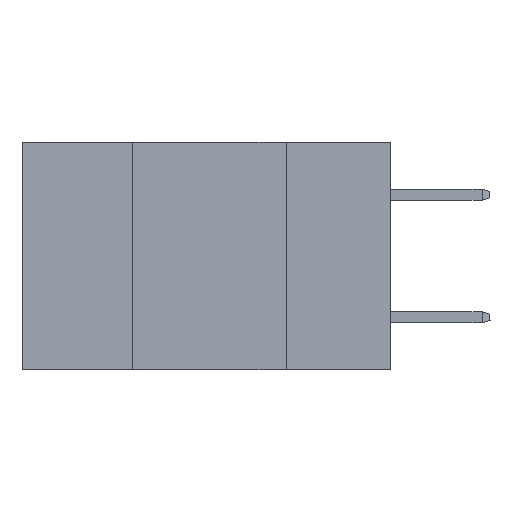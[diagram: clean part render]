
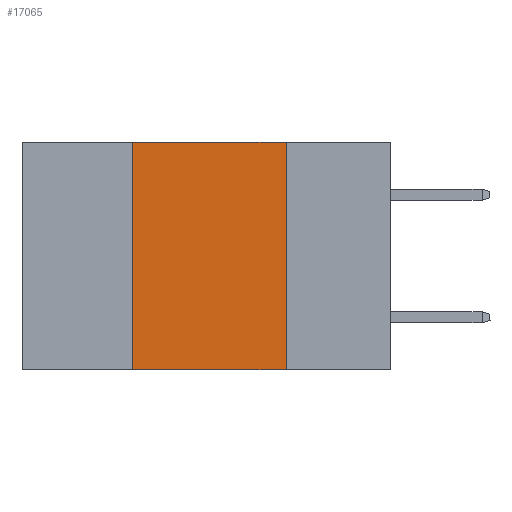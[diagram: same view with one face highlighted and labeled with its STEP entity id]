
A CAD part, left-side view. The second image highlights one B-rep face of the part: STEP entity #17065.
In plain terms, the highlighted planar face has unit normal (-1, 0, 0).
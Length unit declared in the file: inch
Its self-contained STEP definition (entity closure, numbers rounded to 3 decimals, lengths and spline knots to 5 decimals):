
#705 = EDGE_CURVE ( 'NONE', #16371, #19525, #12678, .T. ) ;
#773 = EDGE_CURVE ( 'NONE', #7617, #10101, #20423, .T. ) ;
#986 = DIRECTION ( 'NONE',  ( 0., -1., 0. ) ) ;
#1104 = ORIENTED_EDGE ( 'NONE', *, *, #20048, .F. ) ;
#1252 = VECTOR ( 'NONE', #986, 39.37008 ) ;
#1673 = CARTESIAN_POINT ( 'NONE',  ( 0., 0.6, -0.37 ) ) ;
#3305 = VECTOR ( 'NONE', #12870, 39.37008 ) ;
#3714 = CARTESIAN_POINT ( 'NONE',  ( 0., 0.6, 0. ) ) ;
#4574 = VECTOR ( 'NONE', #19453, 39.37008 ) ;
#4777 = FACE_OUTER_BOUND ( 'NONE', #10656, .T. ) ;
#5422 = DIRECTION ( 'NONE',  ( 0., 0., -1. ) ) ;
#7617 = VERTEX_POINT ( 'NONE', #8149 ) ;
#7718 = LINE ( 'NONE', #26572, #16099 ) ;
#7779 = ORIENTED_EDGE ( 'NONE', *, *, #705, .F. ) ;
#8149 = CARTESIAN_POINT ( 'NONE',  ( 0., 0.42, -0.37 ) ) ;
#8180 = CARTESIAN_POINT ( 'NONE',  ( 0., 0.17, 0. ) ) ;
#8745 = AXIS2_PLACEMENT_3D ( 'NONE', #3714, #10042, #20857 ) ;
#9010 = LINE ( 'NONE', #23450, #3305 ) ;
#9023 = CARTESIAN_POINT ( 'NONE',  ( 0., 0.42, 0. ) ) ;
#10042 = DIRECTION ( 'NONE',  ( 1., 0., 0. ) ) ;
#10101 = VERTEX_POINT ( 'NONE', #25231 ) ;
#10339 = ORIENTED_EDGE ( 'NONE', *, *, #773, .T. ) ;
#10444 = EDGE_CURVE ( 'NONE', #19525, #10101, #7718, .T. ) ;
#10656 = EDGE_LOOP ( 'NONE', ( #11069, #7779, #1104, #10339 ) ) ;
#11069 = ORIENTED_EDGE ( 'NONE', *, *, #10444, .F. ) ;
#11804 = CARTESIAN_POINT ( 'NONE',  ( 0., 0.6, 0. ) ) ;
#12678 = LINE ( 'NONE', #11804, #1252 ) ;
#12870 = DIRECTION ( 'NONE',  ( 0., 0., 1. ) ) ;
#16099 = VECTOR ( 'NONE', #5422, 39.37008 ) ;
#16371 = VERTEX_POINT ( 'NONE', #9023 ) ;
#16568 = PLANE ( 'NONE',  #8745 ) ;
#17065 = ADVANCED_FACE ( 'NONE', ( #4777 ), #16568, .F. ) ;
#19453 = DIRECTION ( 'NONE',  ( 0., -1., 0. ) ) ;
#19525 = VERTEX_POINT ( 'NONE', #8180 ) ;
#20048 = EDGE_CURVE ( 'NONE', #7617, #16371, #9010, .T. ) ;
#20423 = LINE ( 'NONE', #1673, #4574 ) ;
#20857 = DIRECTION ( 'NONE',  ( 0., 0., -1. ) ) ;
#23450 = CARTESIAN_POINT ( 'NONE',  ( 0., 0.42, 0. ) ) ;
#25231 = CARTESIAN_POINT ( 'NONE',  ( 0., 0.17, -0.37 ) ) ;
#26572 = CARTESIAN_POINT ( 'NONE',  ( 0., 0.17, 0. ) ) ;
